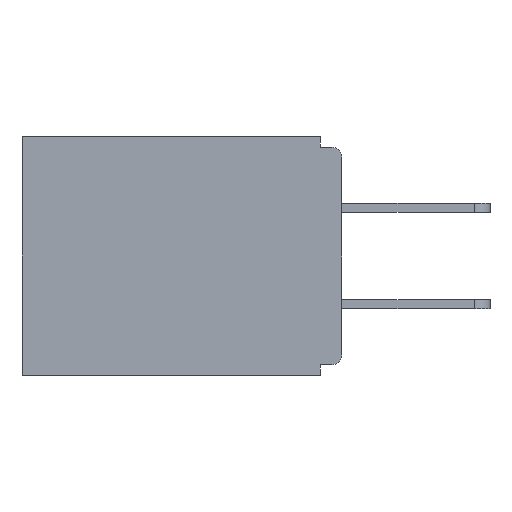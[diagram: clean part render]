
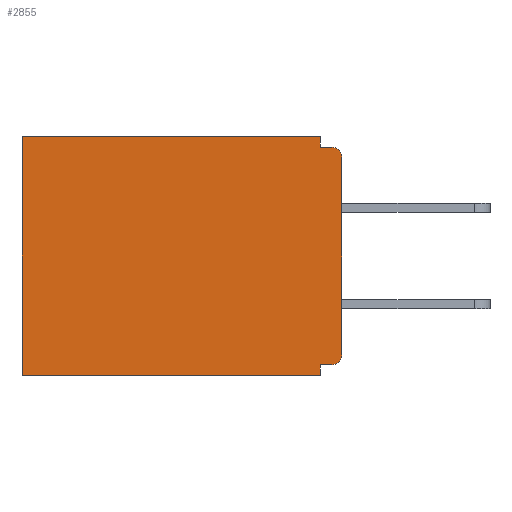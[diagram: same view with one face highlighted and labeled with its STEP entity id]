
A CAD part, left-side view. The second image highlights one B-rep face of the part: STEP entity #2855.
In plain terms, the highlighted planar face has unit normal (-1, 0, 0).
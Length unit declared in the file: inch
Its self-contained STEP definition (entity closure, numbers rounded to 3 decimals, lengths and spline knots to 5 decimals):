
#356 = VECTOR ( 'NONE', #6856, 39.37008 ) ;
#500 = VECTOR ( 'NONE', #1056, 39.37008 ) ;
#1025 = VECTOR ( 'NONE', #17856, 39.37008 ) ;
#1056 = DIRECTION ( 'NONE',  ( 0., 1., 0. ) ) ;
#1344 = VERTEX_POINT ( 'NONE', #9584 ) ;
#2191 = LINE ( 'NONE', #8842, #356 ) ;
#2226 = EDGE_CURVE ( 'NONE', #6172, #3630, #9292, .T. ) ;
#2855 = ADVANCED_FACE ( 'NONE', ( #7152 ), #15457, .F. ) ;
#3226 = CARTESIAN_POINT ( 'NONE',  ( 0.298, 0.015, -0.03 ) ) ;
#3302 = DIRECTION ( 'NONE',  ( -1., 0., 0. ) ) ;
#3345 = LINE ( 'NONE', #10563, #15044 ) ;
#3443 = VERTEX_POINT ( 'NONE', #23654 ) ;
#3630 = VERTEX_POINT ( 'NONE', #16859 ) ;
#3980 = DIRECTION ( 'NONE',  ( 0., 0., -1. ) ) ;
#4460 = CARTESIAN_POINT ( 'NONE',  ( 0.298, 0.46, 0. ) ) ;
#4780 = EDGE_CURVE ( 'NONE', #19558, #23677, #11587, .T. ) ;
#5048 = CARTESIAN_POINT ( 'NONE',  ( 0.298, 0.46, -0.343 ) ) ;
#5201 = EDGE_CURVE ( 'NONE', #3443, #6786, #7626, .T. ) ;
#5668 = CARTESIAN_POINT ( 'NONE',  ( 0.298, 0., -0.313 ) ) ;
#5781 = VERTEX_POINT ( 'NONE', #23567 ) ;
#6091 = AXIS2_PLACEMENT_3D ( 'NONE', #15700, #23451, #3980 ) ;
#6172 = VERTEX_POINT ( 'NONE', #10709 ) ;
#6189 = CARTESIAN_POINT ( 'NONE',  ( 0.298, 0.031, -0.343 ) ) ;
#6304 = EDGE_CURVE ( 'NONE', #5781, #3630, #16884, .T. ) ;
#6540 = VERTEX_POINT ( 'NONE', #22957 ) ;
#6651 = LINE ( 'NONE', #18948, #14165 ) ;
#6786 = VERTEX_POINT ( 'NONE', #5048 ) ;
#6856 = DIRECTION ( 'NONE',  ( 0., 1., 0. ) ) ;
#7048 = CARTESIAN_POINT ( 'NONE',  ( 0.298, 0., -0.343 ) ) ;
#7118 = ORIENTED_EDGE ( 'NONE', *, *, #18401, .T. ) ;
#7152 = FACE_OUTER_BOUND ( 'NONE', #17738, .T. ) ;
#7346 = EDGE_CURVE ( 'NONE', #1344, #20273, #6651, .T. ) ;
#7592 = EDGE_CURVE ( 'NONE', #1344, #6172, #18029, .T. ) ;
#7626 = LINE ( 'NONE', #7048, #500 ) ;
#8276 = ORIENTED_EDGE ( 'NONE', *, *, #14555, .F. ) ;
#8581 = ORIENTED_EDGE ( 'NONE', *, *, #7346, .T. ) ;
#8736 = ORIENTED_EDGE ( 'NONE', *, *, #5201, .F. ) ;
#8756 = DIRECTION ( 'NONE',  ( 0., 0., -1. ) ) ;
#8842 = CARTESIAN_POINT ( 'NONE',  ( 0.298, 0., -0.328 ) ) ;
#9292 = LINE ( 'NONE', #22642, #13209 ) ;
#9584 = CARTESIAN_POINT ( 'NONE',  ( 0.298, 0.031, 0. ) ) ;
#9885 = CARTESIAN_POINT ( 'NONE',  ( 0.298, 0.46, 0. ) ) ;
#9931 = ORIENTED_EDGE ( 'NONE', *, *, #13089, .F. ) ;
#10563 = CARTESIAN_POINT ( 'NONE',  ( 0.298, 0., 0. ) ) ;
#10709 = CARTESIAN_POINT ( 'NONE',  ( 0.298, 0.031, -0.015 ) ) ;
#11587 = CIRCLE ( 'NONE', #19455, 0.015 ) ;
#12049 = DIRECTION ( 'NONE',  ( 0., 0., -1. ) ) ;
#12180 = DIRECTION ( 'NONE',  ( 0., 0., -1. ) ) ;
#12639 = ORIENTED_EDGE ( 'NONE', *, *, #7592, .F. ) ;
#13089 = EDGE_CURVE ( 'NONE', #6540, #3443, #24798, .T. ) ;
#13209 = VECTOR ( 'NONE', #24672, 39.37008 ) ;
#14165 = VECTOR ( 'NONE', #20703, 39.37008 ) ;
#14229 = LINE ( 'NONE', #4460, #1025 ) ;
#14534 = EDGE_CURVE ( 'NONE', #19558, #6540, #2191, .T. ) ;
#14555 = EDGE_CURVE ( 'NONE', #5781, #23677, #3345, .T. ) ;
#14951 = ORIENTED_EDGE ( 'NONE', *, *, #14534, .F. ) ;
#15037 = VECTOR ( 'NONE', #12049, 39.37008 ) ;
#15044 = VECTOR ( 'NONE', #8756, 39.37008 ) ;
#15111 = ORIENTED_EDGE ( 'NONE', *, *, #6304, .T. ) ;
#15387 = CARTESIAN_POINT ( 'NONE',  ( 0.298, 0.015, -0.328 ) ) ;
#15457 = PLANE ( 'NONE',  #6091 ) ;
#15700 = CARTESIAN_POINT ( 'NONE',  ( 0.298, 0., 0. ) ) ;
#15779 = CARTESIAN_POINT ( 'NONE',  ( 0.298, 0.031, -0.343 ) ) ;
#16859 = CARTESIAN_POINT ( 'NONE',  ( 0.298, 0.015, -0.015 ) ) ;
#16884 = CIRCLE ( 'NONE', #21409, 0.015 ) ;
#17738 = EDGE_LOOP ( 'NONE', ( #15111, #18668, #12639, #8581, #7118, #8736, #9931, #14951, #19963, #8276 ) ) ;
#17856 = DIRECTION ( 'NONE',  ( 0., 0., -1. ) ) ;
#18029 = LINE ( 'NONE', #6189, #15037 ) ;
#18401 = EDGE_CURVE ( 'NONE', #20273, #6786, #14229, .T. ) ;
#18668 = ORIENTED_EDGE ( 'NONE', *, *, #2226, .F. ) ;
#18948 = CARTESIAN_POINT ( 'NONE',  ( 0.298, 0., 0. ) ) ;
#19455 = AXIS2_PLACEMENT_3D ( 'NONE', #19807, #21755, #12180 ) ;
#19558 = VERTEX_POINT ( 'NONE', #15387 ) ;
#19807 = CARTESIAN_POINT ( 'NONE',  ( 0.298, 0.015, -0.313 ) ) ;
#19963 = ORIENTED_EDGE ( 'NONE', *, *, #4780, .T. ) ;
#20273 = VERTEX_POINT ( 'NONE', #9885 ) ;
#20703 = DIRECTION ( 'NONE',  ( 0., 1., 0. ) ) ;
#21409 = AXIS2_PLACEMENT_3D ( 'NONE', #3226, #3302, #22368 ) ;
#21755 = DIRECTION ( 'NONE',  ( -1., 0., 0. ) ) ;
#22368 = DIRECTION ( 'NONE',  ( 0., 0., -1. ) ) ;
#22642 = CARTESIAN_POINT ( 'NONE',  ( 0.298, 0., -0.015 ) ) ;
#22957 = CARTESIAN_POINT ( 'NONE',  ( 0.298, 0.031, -0.328 ) ) ;
#23451 = DIRECTION ( 'NONE',  ( 1., 0., 0. ) ) ;
#23529 = DIRECTION ( 'NONE',  ( 0., 0., -1. ) ) ;
#23567 = CARTESIAN_POINT ( 'NONE',  ( 0.298, 0., -0.03 ) ) ;
#23568 = VECTOR ( 'NONE', #23529, 39.37008 ) ;
#23654 = CARTESIAN_POINT ( 'NONE',  ( 0.298, 0.031, -0.343 ) ) ;
#23677 = VERTEX_POINT ( 'NONE', #5668 ) ;
#24672 = DIRECTION ( 'NONE',  ( 0., -1., 0. ) ) ;
#24798 = LINE ( 'NONE', #15779, #23568 ) ;
